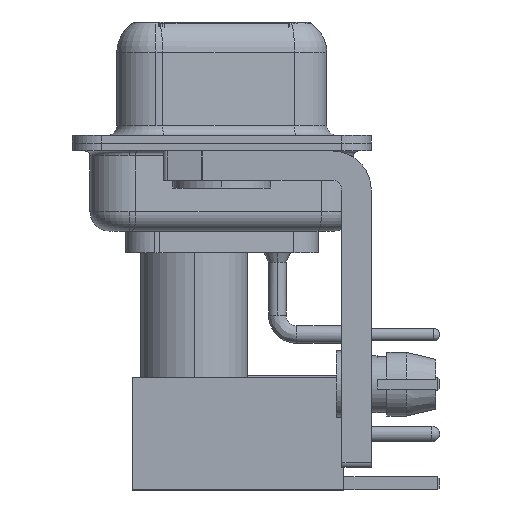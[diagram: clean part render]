
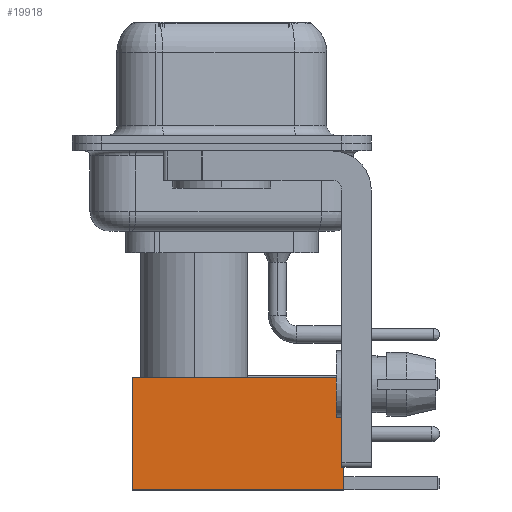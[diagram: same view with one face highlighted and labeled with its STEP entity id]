
A CAD part, left-side view. The second image highlights one B-rep face of the part: STEP entity #19918.
In plain terms, the highlighted face is planar.
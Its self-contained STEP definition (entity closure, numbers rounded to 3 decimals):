
#1126 = EDGE_CURVE ( 'NONE', #17728, #5180, #32146, .T. ) ;
#1147 = CARTESIAN_POINT ( 'NONE',  ( 0., 2.875, 0. ) ) ;
#1649 = VECTOR ( 'NONE', #10125, 1000. ) ;
#3090 = CARTESIAN_POINT ( 'NONE',  ( 2.875, 2.875, 0. ) ) ;
#4838 = AXIS2_PLACEMENT_3D ( 'NONE', #8866, #28571, #25678 ) ;
#4867 = DIRECTION ( 'NONE',  ( -1., 0., 0. ) ) ;
#5180 = VERTEX_POINT ( 'NONE', #32170 ) ;
#7741 = CARTESIAN_POINT ( 'NONE',  ( 0., 2.875, 10.82 ) ) ;
#8866 = CARTESIAN_POINT ( 'NONE',  ( 2.875, 2.875, 0. ) ) ;
#9138 = CARTESIAN_POINT ( 'NONE',  ( 2.875, 2.875, 0. ) ) ;
#10125 = DIRECTION ( 'NONE',  ( 0., 0., -1. ) ) ;
#10299 = LINE ( 'NONE', #29804, #1649 ) ;
#11629 = EDGE_CURVE ( 'NONE', #26064, #26298, #31495, .T. ) ;
#12015 = CARTESIAN_POINT ( 'NONE',  ( 2.875, 2.875, 10.82 ) ) ;
#12163 = ORIENTED_EDGE ( 'NONE', *, *, #14086, .F. ) ;
#13570 = ORIENTED_EDGE ( 'NONE', *, *, #11629, .T. ) ;
#14086 = EDGE_CURVE ( 'NONE', #5180, #26298, #10299, .T. ) ;
#16542 = EDGE_LOOP ( 'NONE', ( #27114, #13570, #12163, #19504 ) ) ;
#16984 = PLANE ( 'NONE',  #4838 ) ;
#17728 = VERTEX_POINT ( 'NONE', #12015 ) ;
#18102 = DIRECTION ( 'NONE',  ( -1., 0., 0. ) ) ;
#19504 = ORIENTED_EDGE ( 'NONE', *, *, #1126, .F. ) ;
#19918 = ADVANCED_FACE ( 'NONE', ( #22592 ), #16984, .T. ) ;
#22592 = FACE_OUTER_BOUND ( 'NONE', #16542, .T. ) ;
#22685 = DIRECTION ( 'NONE',  ( 0., 0., -1. ) ) ;
#22849 = VECTOR ( 'NONE', #18102, 1000. ) ;
#23480 = CARTESIAN_POINT ( 'NONE',  ( -2.875, 2.875, 0. ) ) ;
#25678 = DIRECTION ( 'NONE',  ( 0., 0., 1. ) ) ;
#26064 = VERTEX_POINT ( 'NONE', #3090 ) ;
#26298 = VERTEX_POINT ( 'NONE', #23480 ) ;
#27114 = ORIENTED_EDGE ( 'NONE', *, *, #30371, .T. ) ;
#28002 = VECTOR ( 'NONE', #4867, 1000. ) ;
#28571 = DIRECTION ( 'NONE',  ( 0., 1., 0. ) ) ;
#29804 = CARTESIAN_POINT ( 'NONE',  ( -2.875, 2.875, 0. ) ) ;
#30371 = EDGE_CURVE ( 'NONE', #17728, #26064, #31717, .T. ) ;
#31495 = LINE ( 'NONE', #1147, #22849 ) ;
#31717 = LINE ( 'NONE', #9138, #34755 ) ;
#32146 = LINE ( 'NONE', #7741, #28002 ) ;
#32170 = CARTESIAN_POINT ( 'NONE',  ( -2.875, 2.875, 10.82 ) ) ;
#34755 = VECTOR ( 'NONE', #22685, 1000. ) ;
